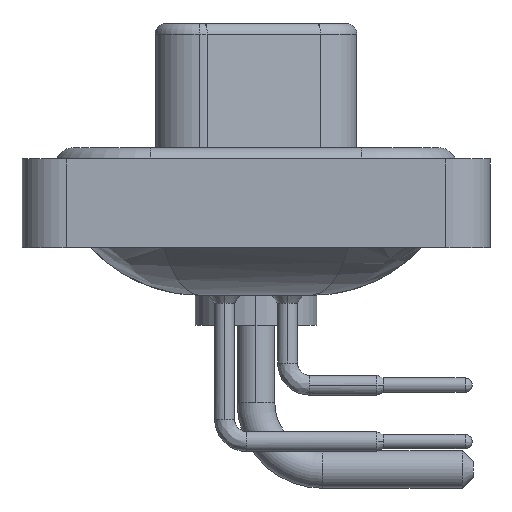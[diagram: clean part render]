
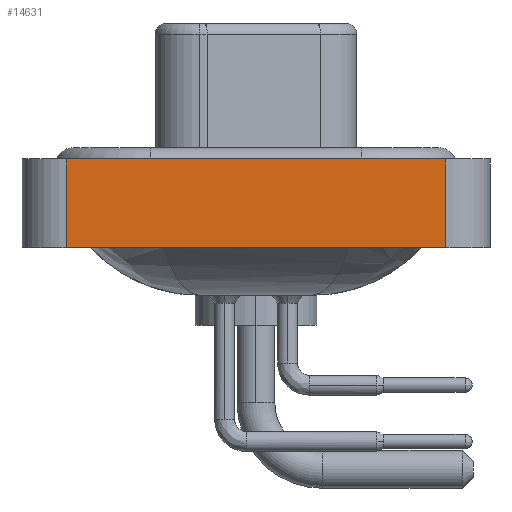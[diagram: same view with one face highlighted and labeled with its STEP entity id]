
A CAD part, left-side view. The second image highlights one B-rep face of the part: STEP entity #14631.
In plain terms, the highlighted planar face has unit normal (-1, 0, 0).
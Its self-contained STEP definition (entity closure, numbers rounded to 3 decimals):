
#327 = AXIS2_PLACEMENT_3D ( 'NONE', #949, #28170, #16662 ) ;
#636 = CARTESIAN_POINT ( 'NONE',  ( -7.35, 8.55, 0.4 ) ) ;
#949 = CARTESIAN_POINT ( 'NONE',  ( -7.35, -8.55, -3.6 ) ) ;
#2231 = VERTEX_POINT ( 'NONE', #636 ) ;
#3372 = VERTEX_POINT ( 'NONE', #22267 ) ;
#4995 = EDGE_CURVE ( 'NONE', #8625, #2231, #16968, .T. ) ;
#5925 = FACE_OUTER_BOUND ( 'NONE', #13450, .T. ) ;
#6636 = EDGE_CURVE ( 'NONE', #8625, #3372, #12304, .T. ) ;
#8036 = VERTEX_POINT ( 'NONE', #8578 ) ;
#8345 = DIRECTION ( 'NONE',  ( 0., -1., 0. ) ) ;
#8578 = CARTESIAN_POINT ( 'NONE',  ( -7.35, -8.55, 0.4 ) ) ;
#8625 = VERTEX_POINT ( 'NONE', #16148 ) ;
#10372 = DIRECTION ( 'NONE',  ( 0., -1., 0. ) ) ;
#11287 = LINE ( 'NONE', #18016, #13044 ) ;
#12304 = LINE ( 'NONE', #19192, #26166 ) ;
#12861 = VECTOR ( 'NONE', #24935, 1000. ) ;
#13044 = VECTOR ( 'NONE', #8345, 1000. ) ;
#13093 = DIRECTION ( 'NONE',  ( 0., 0., 1. ) ) ;
#13123 = ORIENTED_EDGE ( 'NONE', *, *, #23272, .T. ) ;
#13450 = EDGE_LOOP ( 'NONE', ( #13123, #18580, #18305, #19954 ) ) ;
#14563 = PLANE ( 'NONE',  #327 ) ;
#14631 = ADVANCED_FACE ( 'NONE', ( #5925 ), #14563, .T. ) ;
#16148 = CARTESIAN_POINT ( 'NONE',  ( -7.35, 8.55, -3.6 ) ) ;
#16662 = DIRECTION ( 'NONE',  ( 0., 0., 1. ) ) ;
#16968 = LINE ( 'NONE', #19688, #26934 ) ;
#18016 = CARTESIAN_POINT ( 'NONE',  ( -7.35, -8.55, 0.4 ) ) ;
#18305 = ORIENTED_EDGE ( 'NONE', *, *, #4995, .F. ) ;
#18580 = ORIENTED_EDGE ( 'NONE', *, *, #24958, .F. ) ;
#19192 = CARTESIAN_POINT ( 'NONE',  ( -7.35, -8.55, -3.6 ) ) ;
#19688 = CARTESIAN_POINT ( 'NONE',  ( -7.35, 8.55, -3.6 ) ) ;
#19954 = ORIENTED_EDGE ( 'NONE', *, *, #6636, .T. ) ;
#20615 = CARTESIAN_POINT ( 'NONE',  ( -7.35, -8.55, -3.6 ) ) ;
#22267 = CARTESIAN_POINT ( 'NONE',  ( -7.35, -8.55, -3.6 ) ) ;
#23272 = EDGE_CURVE ( 'NONE', #3372, #8036, #25080, .T. ) ;
#24935 = DIRECTION ( 'NONE',  ( 0., 0., 1. ) ) ;
#24958 = EDGE_CURVE ( 'NONE', #2231, #8036, #11287, .T. ) ;
#25080 = LINE ( 'NONE', #20615, #12861 ) ;
#26166 = VECTOR ( 'NONE', #10372, 1000. ) ;
#26934 = VECTOR ( 'NONE', #13093, 1000. ) ;
#28170 = DIRECTION ( 'NONE',  ( -1., 0., 0. ) ) ;
